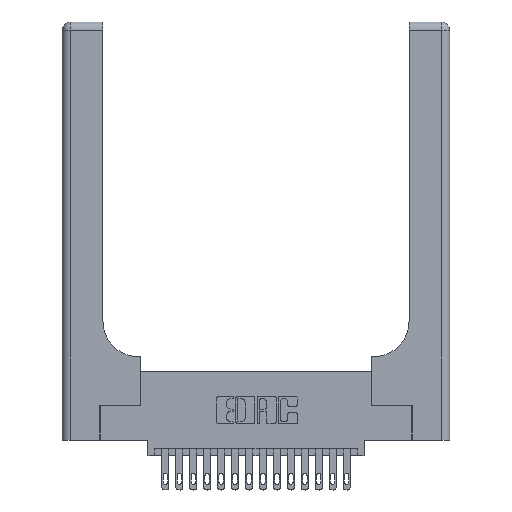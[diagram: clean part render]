
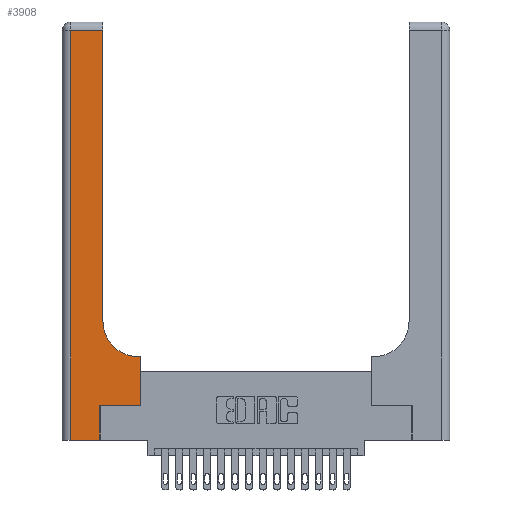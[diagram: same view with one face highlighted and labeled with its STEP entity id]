
A CAD part, top view. The second image highlights one B-rep face of the part: STEP entity #3908.
In plain terms, the highlighted planar face has unit normal (0, 0, 1).
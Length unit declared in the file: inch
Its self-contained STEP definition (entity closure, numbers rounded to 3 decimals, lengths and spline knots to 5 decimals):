
#112 = DIRECTION ( 'NONE',  ( 1., 0., 0. ) ) ;
#334 = LINE ( 'NONE', #16511, #2504 ) ;
#586 = ORIENTED_EDGE ( 'NONE', *, *, #10622, .T. ) ;
#1665 = EDGE_CURVE ( 'NONE', #19798, #12268, #6470, .T. ) ;
#2504 = VECTOR ( 'NONE', #17814, 39.37008 ) ;
#2683 = EDGE_CURVE ( 'NONE', #4318, #15970, #18466, .T. ) ;
#2880 = CARTESIAN_POINT ( 'NONE',  ( 0., 2.94, 0.37 ) ) ;
#2888 = FACE_OUTER_BOUND ( 'NONE', #14027, .T. ) ;
#3114 = CARTESIAN_POINT ( 'NONE',  ( 0.06, 3., 0.37 ) ) ;
#3908 = ADVANCED_FACE ( 'NONE', ( #2888 ), #14960, .F. ) ;
#4160 = VERTEX_POINT ( 'NONE', #9623 ) ;
#4318 = VERTEX_POINT ( 'NONE', #9885 ) ;
#4415 = CIRCLE ( 'NONE', #7642, 0.25 ) ;
#4657 = ORIENTED_EDGE ( 'NONE', *, *, #9486, .T. ) ;
#4867 = CARTESIAN_POINT ( 'NONE',  ( 0., 0., 0.37 ) ) ;
#4915 = EDGE_CURVE ( 'NONE', #12527, #4318, #5747, .T. ) ;
#5232 = ORIENTED_EDGE ( 'NONE', *, *, #4915, .T. ) ;
#5586 = VECTOR ( 'NONE', #15716, 39.37008 ) ;
#5747 = LINE ( 'NONE', #16517, #15450 ) ;
#5811 = CARTESIAN_POINT ( 'NONE',  ( 0.06, 2.94, 0.37 ) ) ;
#5894 = LINE ( 'NONE', #4867, #8336 ) ;
#6157 = CARTESIAN_POINT ( 'NONE',  ( 0.2915, 3., 0.37 ) ) ;
#6334 = ORIENTED_EDGE ( 'NONE', *, *, #16407, .T. ) ;
#6362 = VERTEX_POINT ( 'NONE', #10232 ) ;
#6470 = LINE ( 'NONE', #11235, #12783 ) ;
#7160 = DIRECTION ( 'NONE',  ( 0., 1., 0. ) ) ;
#7642 = AXIS2_PLACEMENT_3D ( 'NONE', #18623, #15379, #112 ) ;
#7935 = EDGE_CURVE ( 'NONE', #18219, #12527, #5894, .T. ) ;
#8049 = CARTESIAN_POINT ( 'NONE',  ( 0.269, 0., 0.37 ) ) ;
#8171 = DIRECTION ( 'NONE',  ( -1., 0., 0. ) ) ;
#8336 = VECTOR ( 'NONE', #11561, 39.37008 ) ;
#8821 = EDGE_CURVE ( 'NONE', #15970, #19798, #334, .T. ) ;
#9085 = VECTOR ( 'NONE', #13867, 39.37008 ) ;
#9486 = EDGE_CURVE ( 'NONE', #4160, #6362, #9860, .T. ) ;
#9623 = CARTESIAN_POINT ( 'NONE',  ( 0.2915, 0.85, 0.37 ) ) ;
#9756 = VECTOR ( 'NONE', #11288, 39.37008 ) ;
#9860 = LINE ( 'NONE', #6157, #11508 ) ;
#9885 = CARTESIAN_POINT ( 'NONE',  ( 0.269, 0.25, 0.37 ) ) ;
#10232 = CARTESIAN_POINT ( 'NONE',  ( 0.2915, 2.94, 0.37 ) ) ;
#10380 = AXIS2_PLACEMENT_3D ( 'NONE', #16528, #12116, #12314 ) ;
#10622 = EDGE_CURVE ( 'NONE', #6362, #15899, #17302, .T. ) ;
#11235 = CARTESIAN_POINT ( 'NONE',  ( 0.2915, 0.6, 0.37 ) ) ;
#11288 = DIRECTION ( 'NONE',  ( 1., 0., 0. ) ) ;
#11508 = VECTOR ( 'NONE', #19977, 39.37008 ) ;
#11561 = DIRECTION ( 'NONE',  ( 1., 0., 0. ) ) ;
#12116 = DIRECTION ( 'NONE',  ( 0., 0., -1. ) ) ;
#12222 = CARTESIAN_POINT ( 'NONE',  ( 0.06, 0., 0.37 ) ) ;
#12268 = VERTEX_POINT ( 'NONE', #16599 ) ;
#12314 = DIRECTION ( 'NONE',  ( -1., 0., 0. ) ) ;
#12527 = VERTEX_POINT ( 'NONE', #8049 ) ;
#12783 = VECTOR ( 'NONE', #8171, 39.37008 ) ;
#12854 = ORIENTED_EDGE ( 'NONE', *, *, #2683, .T. ) ;
#12941 = CARTESIAN_POINT ( 'NONE',  ( 0.5585, 0.6, 0.37 ) ) ;
#13867 = DIRECTION ( 'NONE',  ( -1., 0., 0. ) ) ;
#14027 = EDGE_LOOP ( 'NONE', ( #4657, #586, #18628, #19591, #5232, #12854, #17211, #18571, #6334 ) ) ;
#14322 = LINE ( 'NONE', #3114, #5586 ) ;
#14471 = CARTESIAN_POINT ( 'NONE',  ( 0.269, 0.25, 0.37 ) ) ;
#14960 = PLANE ( 'NONE',  #10380 ) ;
#15379 = DIRECTION ( 'NONE',  ( 0., 0., -1. ) ) ;
#15450 = VECTOR ( 'NONE', #7160, 39.37008 ) ;
#15716 = DIRECTION ( 'NONE',  ( 0., -1., 0. ) ) ;
#15899 = VERTEX_POINT ( 'NONE', #5811 ) ;
#15970 = VERTEX_POINT ( 'NONE', #19909 ) ;
#16407 = EDGE_CURVE ( 'NONE', #12268, #4160, #4415, .T. ) ;
#16511 = CARTESIAN_POINT ( 'NONE',  ( 0.5585, 0.25, 0.37 ) ) ;
#16517 = CARTESIAN_POINT ( 'NONE',  ( 0.269, 0., 0.37 ) ) ;
#16528 = CARTESIAN_POINT ( 'NONE',  ( 0., 3., 0.37 ) ) ;
#16599 = CARTESIAN_POINT ( 'NONE',  ( 0.5415, 0.6, 0.37 ) ) ;
#17211 = ORIENTED_EDGE ( 'NONE', *, *, #8821, .T. ) ;
#17302 = LINE ( 'NONE', #2880, #9085 ) ;
#17814 = DIRECTION ( 'NONE',  ( 0., 1., 0. ) ) ;
#18219 = VERTEX_POINT ( 'NONE', #12222 ) ;
#18363 = EDGE_CURVE ( 'NONE', #15899, #18219, #14322, .T. ) ;
#18466 = LINE ( 'NONE', #14471, #9756 ) ;
#18571 = ORIENTED_EDGE ( 'NONE', *, *, #1665, .T. ) ;
#18623 = CARTESIAN_POINT ( 'NONE',  ( 0.5415, 0.85, 0.37 ) ) ;
#18628 = ORIENTED_EDGE ( 'NONE', *, *, #18363, .T. ) ;
#19591 = ORIENTED_EDGE ( 'NONE', *, *, #7935, .T. ) ;
#19798 = VERTEX_POINT ( 'NONE', #12941 ) ;
#19909 = CARTESIAN_POINT ( 'NONE',  ( 0.5585, 0.25, 0.37 ) ) ;
#19977 = DIRECTION ( 'NONE',  ( 0., 1., 0. ) ) ;
